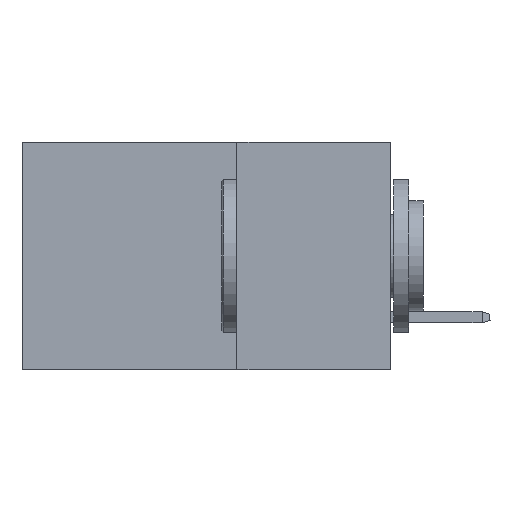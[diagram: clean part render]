
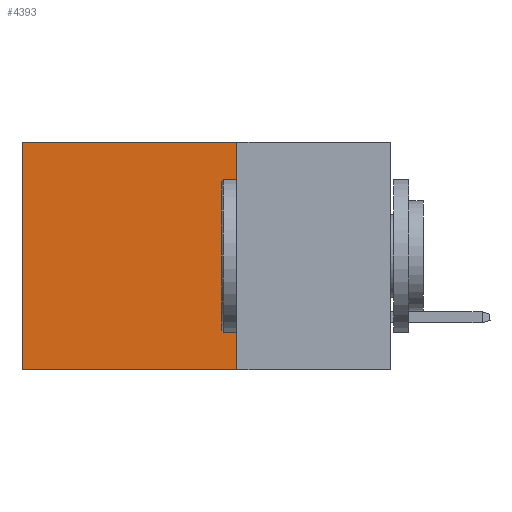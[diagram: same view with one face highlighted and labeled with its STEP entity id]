
A CAD part, left-side view. The second image highlights one B-rep face of the part: STEP entity #4393.
In plain terms, the highlighted planar face has unit normal (-1, 0, 0).
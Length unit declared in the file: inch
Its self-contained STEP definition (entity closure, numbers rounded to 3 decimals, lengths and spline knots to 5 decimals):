
#1133 = CARTESIAN_POINT ( 'NONE',  ( 0.2875, 0.25, 0. ) ) ;
#1597 = ORIENTED_EDGE ( 'NONE', *, *, #4680, .T. ) ;
#3137 = VECTOR ( 'NONE', #16857, 39.37008 ) ;
#3303 = CARTESIAN_POINT ( 'NONE',  ( 0.2875, 0.6, -0.37 ) ) ;
#3684 = FACE_OUTER_BOUND ( 'NONE', #5983, .T. ) ;
#4291 = VERTEX_POINT ( 'NONE', #3303 ) ;
#4349 = VERTEX_POINT ( 'NONE', #1133 ) ;
#4393 = ADVANCED_FACE ( 'NONE', ( #3684 ), #16459, .F. ) ;
#4680 = EDGE_CURVE ( 'NONE', #12859, #4291, #19338, .T. ) ;
#5119 = CARTESIAN_POINT ( 'NONE',  ( 0.2875, 0.6, 0. ) ) ;
#5232 = LINE ( 'NONE', #19033, #9932 ) ;
#5983 = EDGE_LOOP ( 'NONE', ( #1597, #15025, #16499, #7732 ) ) ;
#6110 = CARTESIAN_POINT ( 'NONE',  ( 0.2875, 0.25, 0. ) ) ;
#6620 = LINE ( 'NONE', #12444, #3137 ) ;
#7378 = VECTOR ( 'NONE', #17658, 39.37008 ) ;
#7732 = ORIENTED_EDGE ( 'NONE', *, *, #11633, .T. ) ;
#8810 = CARTESIAN_POINT ( 'NONE',  ( 0.2875, 0.6, 0. ) ) ;
#9029 = CARTESIAN_POINT ( 'NONE',  ( 0.2875, 0.25, -0.37 ) ) ;
#9932 = VECTOR ( 'NONE', #17592, 39.37008 ) ;
#10589 = DIRECTION ( 'NONE',  ( 1., 0., 0. ) ) ;
#11177 = EDGE_CURVE ( 'NONE', #4349, #11876, #6620, .T. ) ;
#11633 = EDGE_CURVE ( 'NONE', #4349, #12859, #17393, .T. ) ;
#11876 = VERTEX_POINT ( 'NONE', #9029 ) ;
#12099 = DIRECTION ( 'NONE',  ( 0., 0., -1. ) ) ;
#12444 = CARTESIAN_POINT ( 'NONE',  ( 0.2875, 0.25, 0. ) ) ;
#12859 = VERTEX_POINT ( 'NONE', #5119 ) ;
#14807 = VECTOR ( 'NONE', #16476, 39.37008 ) ;
#15013 = AXIS2_PLACEMENT_3D ( 'NONE', #6110, #10589, #12099 ) ;
#15025 = ORIENTED_EDGE ( 'NONE', *, *, #17324, .F. ) ;
#16459 = PLANE ( 'NONE',  #15013 ) ;
#16476 = DIRECTION ( 'NONE',  ( 0., 1., 0. ) ) ;
#16499 = ORIENTED_EDGE ( 'NONE', *, *, #11177, .F. ) ;
#16857 = DIRECTION ( 'NONE',  ( 0., 0., -1. ) ) ;
#17324 = EDGE_CURVE ( 'NONE', #11876, #4291, #5232, .T. ) ;
#17393 = LINE ( 'NONE', #17798, #14807 ) ;
#17592 = DIRECTION ( 'NONE',  ( 0., 1., 0. ) ) ;
#17658 = DIRECTION ( 'NONE',  ( 0., 0., -1. ) ) ;
#17798 = CARTESIAN_POINT ( 'NONE',  ( 0.2875, 0.25, 0. ) ) ;
#19033 = CARTESIAN_POINT ( 'NONE',  ( 0.2875, 0.25, -0.37 ) ) ;
#19338 = LINE ( 'NONE', #8810, #7378 ) ;
